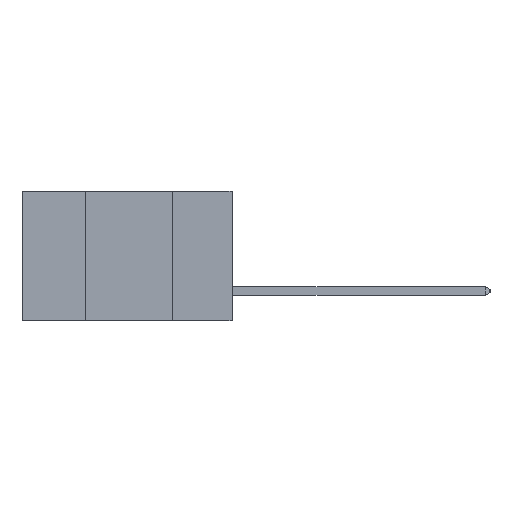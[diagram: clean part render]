
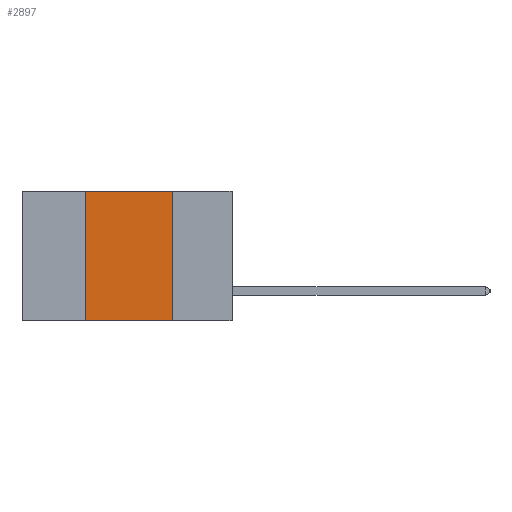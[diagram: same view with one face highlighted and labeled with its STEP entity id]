
A CAD part, left-side view. The second image highlights one B-rep face of the part: STEP entity #2897.
In plain terms, the highlighted planar face has unit normal (-1, 0, 0).
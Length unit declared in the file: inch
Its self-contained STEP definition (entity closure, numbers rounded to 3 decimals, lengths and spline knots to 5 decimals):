
#606 = LINE ( 'NONE', #8052, #5358 ) ;
#1048 = EDGE_CURVE ( 'NONE', #7548, #8599, #606, .T. ) ;
#2897 = ADVANCED_FACE ( 'NONE', ( #19271 ), #9495, .F. ) ;
#3365 = ORIENTED_EDGE ( 'NONE', *, *, #16355, .F. ) ;
#3741 = CARTESIAN_POINT ( 'NONE',  ( 0., 0.17, 0. ) ) ;
#5148 = VERTEX_POINT ( 'NONE', #16866 ) ;
#5358 = VECTOR ( 'NONE', #21560, 39.37008 ) ;
#5405 = AXIS2_PLACEMENT_3D ( 'NONE', #6458, #11383, #16467 ) ;
#5629 = DIRECTION ( 'NONE',  ( 0., -1., 0. ) ) ;
#5718 = VECTOR ( 'NONE', #10674, 39.37008 ) ;
#6458 = CARTESIAN_POINT ( 'NONE',  ( 0., 0.6, 0. ) ) ;
#6756 = CARTESIAN_POINT ( 'NONE',  ( 0., 0.6, -0.37 ) ) ;
#7068 = CARTESIAN_POINT ( 'NONE',  ( 0., 0.42, 0. ) ) ;
#7145 = EDGE_LOOP ( 'NONE', ( #3365, #9969, #15683, #17121 ) ) ;
#7548 = VERTEX_POINT ( 'NONE', #9267 ) ;
#8052 = CARTESIAN_POINT ( 'NONE',  ( 0., 0.6, 0. ) ) ;
#8599 = VERTEX_POINT ( 'NONE', #3741 ) ;
#9267 = CARTESIAN_POINT ( 'NONE',  ( 0., 0.42, 0. ) ) ;
#9495 = PLANE ( 'NONE',  #5405 ) ;
#9969 = ORIENTED_EDGE ( 'NONE', *, *, #1048, .F. ) ;
#10035 = VERTEX_POINT ( 'NONE', #18707 ) ;
#10674 = DIRECTION ( 'NONE',  ( 0., 0., -1. ) ) ;
#11298 = EDGE_CURVE ( 'NONE', #10035, #5148, #18745, .T. ) ;
#11383 = DIRECTION ( 'NONE',  ( 1., 0., 0. ) ) ;
#12190 = VECTOR ( 'NONE', #5629, 39.37008 ) ;
#13547 = VECTOR ( 'NONE', #17067, 39.37008 ) ;
#15683 = ORIENTED_EDGE ( 'NONE', *, *, #17460, .F. ) ;
#16355 = EDGE_CURVE ( 'NONE', #8599, #5148, #20430, .T. ) ;
#16467 = DIRECTION ( 'NONE',  ( 0., 0., -1. ) ) ;
#16866 = CARTESIAN_POINT ( 'NONE',  ( 0., 0.17, -0.37 ) ) ;
#17067 = DIRECTION ( 'NONE',  ( 0., 0., 1. ) ) ;
#17121 = ORIENTED_EDGE ( 'NONE', *, *, #11298, .T. ) ;
#17460 = EDGE_CURVE ( 'NONE', #10035, #7548, #18041, .T. ) ;
#18041 = LINE ( 'NONE', #7068, #13547 ) ;
#18707 = CARTESIAN_POINT ( 'NONE',  ( 0., 0.42, -0.37 ) ) ;
#18745 = LINE ( 'NONE', #6756, #12190 ) ;
#18815 = CARTESIAN_POINT ( 'NONE',  ( 0., 0.17, 0. ) ) ;
#19271 = FACE_OUTER_BOUND ( 'NONE', #7145, .T. ) ;
#20430 = LINE ( 'NONE', #18815, #5718 ) ;
#21560 = DIRECTION ( 'NONE',  ( 0., -1., 0. ) ) ;
